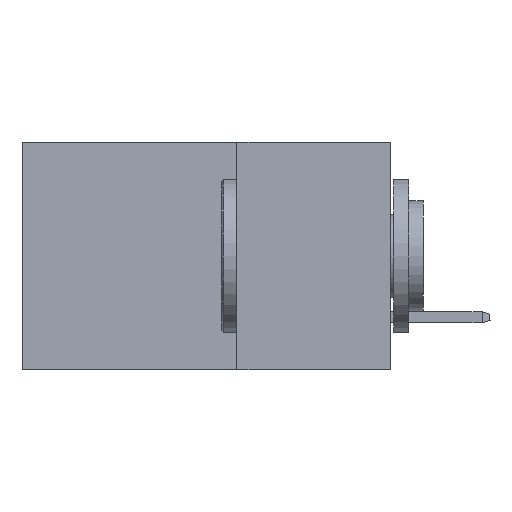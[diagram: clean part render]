
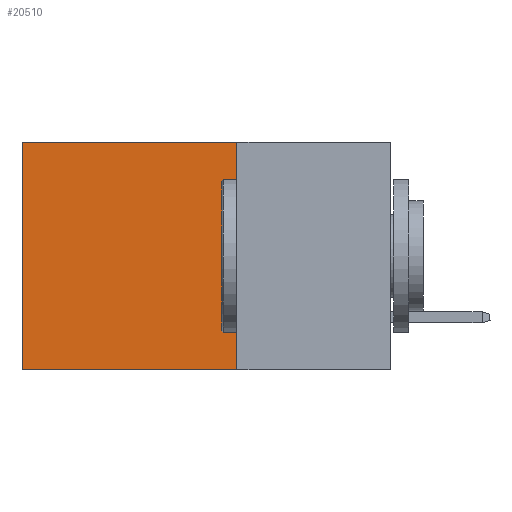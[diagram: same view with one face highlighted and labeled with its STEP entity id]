
A CAD part, left-side view. The second image highlights one B-rep face of the part: STEP entity #20510.
In plain terms, the highlighted planar face has unit normal (-1, 0, 0).
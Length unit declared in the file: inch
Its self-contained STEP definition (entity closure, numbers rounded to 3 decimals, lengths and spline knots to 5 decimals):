
#1 = EDGE_LOOP ( 'NONE', ( #26208, #8122, #5050, #9528 ) ) ;
#1134 = AXIS2_PLACEMENT_3D ( 'NONE', #9303, #17647, #33544 ) ;
#1626 = CARTESIAN_POINT ( 'NONE',  ( 0.2875, 0.25, 0. ) ) ;
#2328 = VECTOR ( 'NONE', #19225, 39.37008 ) ;
#3943 = VECTOR ( 'NONE', #4655, 39.37008 ) ;
#4655 = DIRECTION ( 'NONE',  ( 0., 0., -1. ) ) ;
#5050 = ORIENTED_EDGE ( 'NONE', *, *, #32397, .F. ) ;
#5119 = CARTESIAN_POINT ( 'NONE',  ( 0.2875, 0.25, -0.37 ) ) ;
#5216 = LINE ( 'NONE', #27795, #15367 ) ;
#6125 = DIRECTION ( 'NONE',  ( 0., 0., -1. ) ) ;
#6144 = LINE ( 'NONE', #11014, #2328 ) ;
#7747 = VECTOR ( 'NONE', #6125, 39.37008 ) ;
#8098 = EDGE_CURVE ( 'NONE', #33999, #28678, #5216, .T. ) ;
#8122 = ORIENTED_EDGE ( 'NONE', *, *, #8098, .F. ) ;
#8986 = LINE ( 'NONE', #30190, #7747 ) ;
#9303 = CARTESIAN_POINT ( 'NONE',  ( 0.2875, 0.25, 0. ) ) ;
#9528 = ORIENTED_EDGE ( 'NONE', *, *, #23187, .T. ) ;
#10014 = CARTESIAN_POINT ( 'NONE',  ( 0.2875, 0.6, 0. ) ) ;
#11014 = CARTESIAN_POINT ( 'NONE',  ( 0.2875, 0.25, 0. ) ) ;
#15030 = EDGE_CURVE ( 'NONE', #20047, #28678, #23345, .T. ) ;
#15367 = VECTOR ( 'NONE', #19269, 39.37008 ) ;
#17647 = DIRECTION ( 'NONE',  ( 1., 0., 0. ) ) ;
#19225 = DIRECTION ( 'NONE',  ( 0., 1., 0. ) ) ;
#19269 = DIRECTION ( 'NONE',  ( 0., 1., 0. ) ) ;
#19691 = CARTESIAN_POINT ( 'NONE',  ( 0.2875, 0.6, -0.37 ) ) ;
#20047 = VERTEX_POINT ( 'NONE', #33813 ) ;
#20510 = ADVANCED_FACE ( 'NONE', ( #33435 ), #33664, .F. ) ;
#23187 = EDGE_CURVE ( 'NONE', #23962, #20047, #6144, .T. ) ;
#23345 = LINE ( 'NONE', #10014, #3943 ) ;
#23962 = VERTEX_POINT ( 'NONE', #1626 ) ;
#26208 = ORIENTED_EDGE ( 'NONE', *, *, #15030, .T. ) ;
#27795 = CARTESIAN_POINT ( 'NONE',  ( 0.2875, 0.25, -0.37 ) ) ;
#28678 = VERTEX_POINT ( 'NONE', #19691 ) ;
#30190 = CARTESIAN_POINT ( 'NONE',  ( 0.2875, 0.25, 0. ) ) ;
#32397 = EDGE_CURVE ( 'NONE', #23962, #33999, #8986, .T. ) ;
#33435 = FACE_OUTER_BOUND ( 'NONE', #1, .T. ) ;
#33544 = DIRECTION ( 'NONE',  ( 0., 0., -1. ) ) ;
#33664 = PLANE ( 'NONE',  #1134 ) ;
#33813 = CARTESIAN_POINT ( 'NONE',  ( 0.2875, 0.6, 0. ) ) ;
#33999 = VERTEX_POINT ( 'NONE', #5119 ) ;
